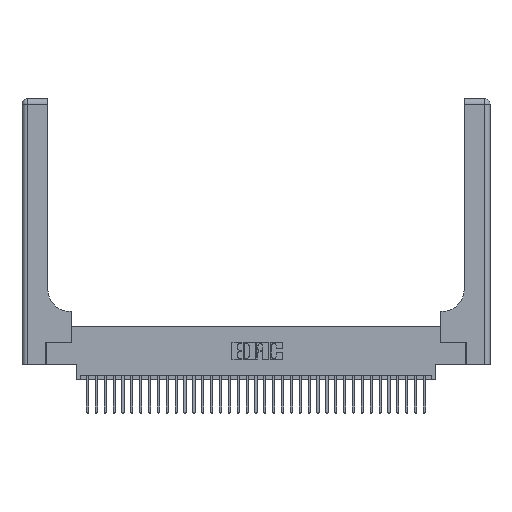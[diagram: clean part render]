
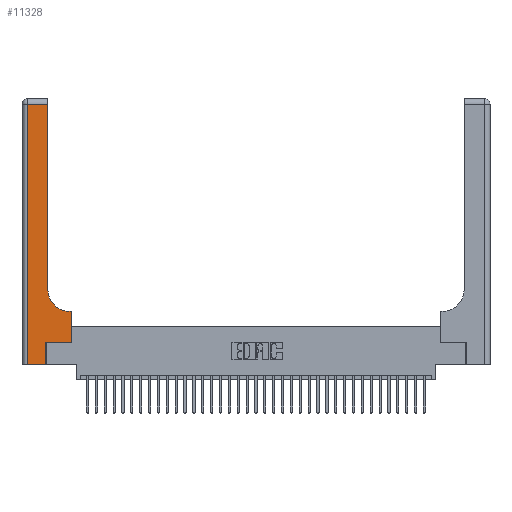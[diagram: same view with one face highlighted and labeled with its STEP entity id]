
A CAD part, top view. The second image highlights one B-rep face of the part: STEP entity #11328.
In plain terms, the highlighted planar face has unit normal (0, 0, 1).
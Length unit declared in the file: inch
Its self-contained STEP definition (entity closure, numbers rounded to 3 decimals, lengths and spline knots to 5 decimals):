
#78 = ORIENTED_EDGE ( 'NONE', *, *, #21073, .T. ) ;
#1568 = CARTESIAN_POINT ( 'NONE',  ( 0., 2.94, 0.37 ) ) ;
#1879 = DIRECTION ( 'NONE',  ( 0., 1., 0. ) ) ;
#2344 = DIRECTION ( 'NONE',  ( 0., 1., 0. ) ) ;
#2638 = CARTESIAN_POINT ( 'NONE',  ( 0.06, 2.94, 0.37 ) ) ;
#3035 = PLANE ( 'NONE',  #12783 ) ;
#3058 = EDGE_CURVE ( 'NONE', #35646, #10659, #12367, .T. ) ;
#3068 = VECTOR ( 'NONE', #29940, 39.37008 ) ;
#3294 = EDGE_CURVE ( 'NONE', #30355, #25282, #33403, .T. ) ;
#4056 = EDGE_CURVE ( 'NONE', #8889, #30355, #17996, .T. ) ;
#4106 = ORIENTED_EDGE ( 'NONE', *, *, #3058, .T. ) ;
#4412 = DIRECTION ( 'NONE',  ( -1., 0., 0. ) ) ;
#4903 = VECTOR ( 'NONE', #1879, 39.37008 ) ;
#5861 = VECTOR ( 'NONE', #29695, 39.37008 ) ;
#5870 = DIRECTION ( 'NONE',  ( -1., 0., 0. ) ) ;
#5881 = CARTESIAN_POINT ( 'NONE',  ( 0.06, 0., 0.37 ) ) ;
#7965 = VECTOR ( 'NONE', #28822, 39.37008 ) ;
#8352 = DIRECTION ( 'NONE',  ( 0., -1., 0. ) ) ;
#8889 = VERTEX_POINT ( 'NONE', #32045 ) ;
#9033 = DIRECTION ( 'NONE',  ( 0., 0., -1. ) ) ;
#9195 = VECTOR ( 'NONE', #27013, 39.37008 ) ;
#9372 = EDGE_LOOP ( 'NONE', ( #29615, #25651, #15963, #33504, #4106, #29608, #78, #11134, #29641 ) ) ;
#9707 = CARTESIAN_POINT ( 'NONE',  ( 0.2915, 2.94, 0.37 ) ) ;
#10227 = EDGE_CURVE ( 'NONE', #10659, #20372, #11467, .T. ) ;
#10659 = VERTEX_POINT ( 'NONE', #22629 ) ;
#11134 = ORIENTED_EDGE ( 'NONE', *, *, #4056, .T. ) ;
#11328 = ADVANCED_FACE ( 'NONE', ( #17149 ), #3035, .F. ) ;
#11386 = CARTESIAN_POINT ( 'NONE',  ( 0., 3., 0.37 ) ) ;
#11467 = LINE ( 'NONE', #14778, #7965 ) ;
#12367 = LINE ( 'NONE', #27093, #4903 ) ;
#12783 = AXIS2_PLACEMENT_3D ( 'NONE', #11386, #22713, #5870 ) ;
#12933 = LINE ( 'NONE', #25199, #33540 ) ;
#13354 = VECTOR ( 'NONE', #2344, 39.37008 ) ;
#14778 = CARTESIAN_POINT ( 'NONE',  ( 0.269, 0.25, 0.37 ) ) ;
#15963 = ORIENTED_EDGE ( 'NONE', *, *, #21591, .T. ) ;
#16050 = EDGE_CURVE ( 'NONE', #25282, #33391, #29200, .T. ) ;
#17149 = FACE_OUTER_BOUND ( 'NONE', #9372, .T. ) ;
#17602 = VERTEX_POINT ( 'NONE', #2638 ) ;
#17996 = LINE ( 'NONE', #27081, #3068 ) ;
#19849 = CARTESIAN_POINT ( 'NONE',  ( 0.269, 0., 0.37 ) ) ;
#20372 = VERTEX_POINT ( 'NONE', #30946 ) ;
#21073 = EDGE_CURVE ( 'NONE', #20372, #8889, #28333, .T. ) ;
#21591 = EDGE_CURVE ( 'NONE', #17602, #28452, #12933, .T. ) ;
#22629 = CARTESIAN_POINT ( 'NONE',  ( 0.269, 0.25, 0.37 ) ) ;
#22713 = DIRECTION ( 'NONE',  ( 0., 0., -1. ) ) ;
#24046 = CARTESIAN_POINT ( 'NONE',  ( 0.2915, 3., 0.37 ) ) ;
#24159 = LINE ( 'NONE', #24218, #9195 ) ;
#24218 = CARTESIAN_POINT ( 'NONE',  ( 0., 0., 0.37 ) ) ;
#25199 = CARTESIAN_POINT ( 'NONE',  ( 0.06, 3., 0.37 ) ) ;
#25282 = VERTEX_POINT ( 'NONE', #33102 ) ;
#25651 = ORIENTED_EDGE ( 'NONE', *, *, #26947, .T. ) ;
#25868 = CARTESIAN_POINT ( 'NONE',  ( 0.5415, 0.85, 0.37 ) ) ;
#26298 = CARTESIAN_POINT ( 'NONE',  ( 0.5415, 0.6, 0.37 ) ) ;
#26947 = EDGE_CURVE ( 'NONE', #33391, #17602, #27868, .T. ) ;
#27013 = DIRECTION ( 'NONE',  ( 1., 0., 0. ) ) ;
#27081 = CARTESIAN_POINT ( 'NONE',  ( 0.2915, 0.6, 0.37 ) ) ;
#27093 = CARTESIAN_POINT ( 'NONE',  ( 0.269, 0., 0.37 ) ) ;
#27868 = LINE ( 'NONE', #1568, #33511 ) ;
#28333 = LINE ( 'NONE', #33655, #13354 ) ;
#28452 = VERTEX_POINT ( 'NONE', #5881 ) ;
#28711 = DIRECTION ( 'NONE',  ( 1., 0., 0. ) ) ;
#28822 = DIRECTION ( 'NONE',  ( 1., 0., 0. ) ) ;
#29200 = LINE ( 'NONE', #24046, #5861 ) ;
#29608 = ORIENTED_EDGE ( 'NONE', *, *, #10227, .T. ) ;
#29615 = ORIENTED_EDGE ( 'NONE', *, *, #16050, .T. ) ;
#29641 = ORIENTED_EDGE ( 'NONE', *, *, #3294, .T. ) ;
#29695 = DIRECTION ( 'NONE',  ( 0., 1., 0. ) ) ;
#29940 = DIRECTION ( 'NONE',  ( -1., 0., 0. ) ) ;
#30355 = VERTEX_POINT ( 'NONE', #26298 ) ;
#30946 = CARTESIAN_POINT ( 'NONE',  ( 0.5585, 0.25, 0.37 ) ) ;
#32045 = CARTESIAN_POINT ( 'NONE',  ( 0.5585, 0.6, 0.37 ) ) ;
#33102 = CARTESIAN_POINT ( 'NONE',  ( 0.2915, 0.85, 0.37 ) ) ;
#33391 = VERTEX_POINT ( 'NONE', #9707 ) ;
#33403 = CIRCLE ( 'NONE', #34483, 0.25 ) ;
#33504 = ORIENTED_EDGE ( 'NONE', *, *, #35316, .T. ) ;
#33511 = VECTOR ( 'NONE', #4412, 39.37008 ) ;
#33540 = VECTOR ( 'NONE', #8352, 39.37008 ) ;
#33655 = CARTESIAN_POINT ( 'NONE',  ( 0.5585, 0.25, 0.37 ) ) ;
#34483 = AXIS2_PLACEMENT_3D ( 'NONE', #25868, #9033, #28711 ) ;
#35316 = EDGE_CURVE ( 'NONE', #28452, #35646, #24159, .T. ) ;
#35646 = VERTEX_POINT ( 'NONE', #19849 ) ;
